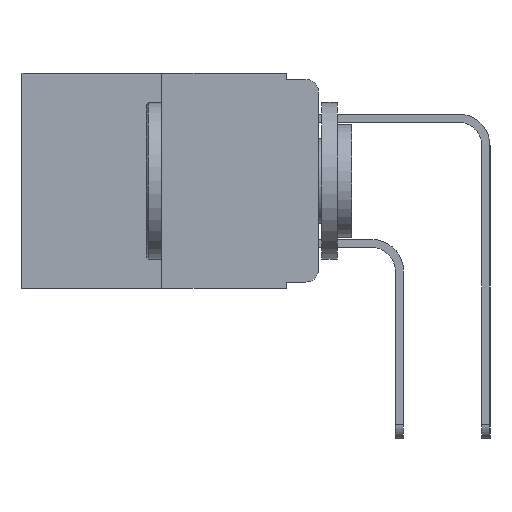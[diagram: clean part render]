
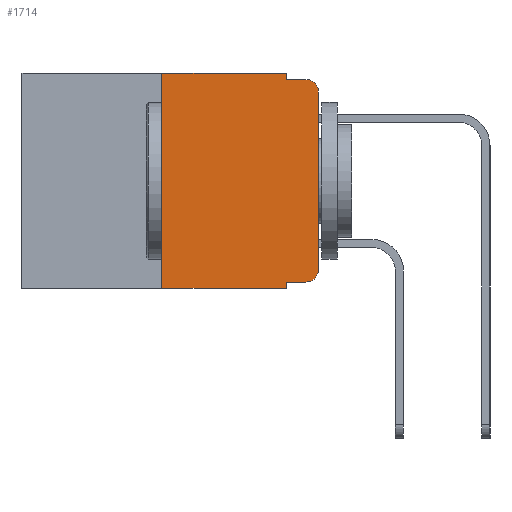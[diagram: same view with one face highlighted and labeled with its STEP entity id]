
A CAD part, left-side view. The second image highlights one B-rep face of the part: STEP entity #1714.
In plain terms, the highlighted planar face has unit normal (-1, 0, 0).
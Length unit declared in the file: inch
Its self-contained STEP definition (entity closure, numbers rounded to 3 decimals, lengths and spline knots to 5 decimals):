
#1017 = VERTEX_POINT ( 'NONE', #15963 ) ;
#1200 = LINE ( 'NONE', #21345, #18734 ) ;
#1714 = ADVANCED_FACE ( 'NONE', ( #17497 ), #11822, .F. ) ;
#1835 = AXIS2_PLACEMENT_3D ( 'NONE', #11015, #10094, #11065 ) ;
#1918 = VERTEX_POINT ( 'NONE', #8275 ) ;
#2695 = VERTEX_POINT ( 'NONE', #4672 ) ;
#2706 = CARTESIAN_POINT ( 'NONE',  ( 0., 0.473, 0. ) ) ;
#2794 = VERTEX_POINT ( 'NONE', #3495 ) ;
#2988 = AXIS2_PLACEMENT_3D ( 'NONE', #6058, #17907, #7817 ) ;
#3069 = CIRCLE ( 'NONE', #2988, 0.02 ) ;
#3096 = EDGE_CURVE ( 'NONE', #1918, #1017, #21475, .T. ) ;
#3413 = LINE ( 'NONE', #7928, #20769 ) ;
#3495 = CARTESIAN_POINT ( 'NONE',  ( 0., 0.051, -0.01 ) ) ;
#3724 = DIRECTION ( 'NONE',  ( 0., -1., 0. ) ) ;
#3997 = LINE ( 'NONE', #19282, #12645 ) ;
#4003 = DIRECTION ( 'NONE',  ( 0., 0., -1. ) ) ;
#4215 = LINE ( 'NONE', #12328, #17250 ) ;
#4513 = DIRECTION ( 'NONE',  ( 0., -1., 0. ) ) ;
#4614 = DIRECTION ( 'NONE',  ( 0., 0., -1. ) ) ;
#4672 = CARTESIAN_POINT ( 'NONE',  ( 0., 0.02, -0.01 ) ) ;
#4783 = ORIENTED_EDGE ( 'NONE', *, *, #11661, .T. ) ;
#4968 = VERTEX_POINT ( 'NONE', #19888 ) ;
#6058 = CARTESIAN_POINT ( 'NONE',  ( 0., 0.02, -0.313 ) ) ;
#6405 = EDGE_CURVE ( 'NONE', #2794, #2695, #3997, .T. ) ;
#6433 = DIRECTION ( 'NONE',  ( 0., 0., -1. ) ) ;
#6610 = CARTESIAN_POINT ( 'NONE',  ( 0., 0.25, 0. ) ) ;
#6652 = ORIENTED_EDGE ( 'NONE', *, *, #21400, .F. ) ;
#7103 = CARTESIAN_POINT ( 'NONE',  ( 0., 0., 0. ) ) ;
#7124 = LINE ( 'NONE', #2706, #15639 ) ;
#7354 = VERTEX_POINT ( 'NONE', #6610 ) ;
#7569 = EDGE_CURVE ( 'NONE', #4968, #2695, #11796, .T. ) ;
#7726 = CARTESIAN_POINT ( 'NONE',  ( 0., 0.02, -0.03 ) ) ;
#7817 = DIRECTION ( 'NONE',  ( 0., 0., -1. ) ) ;
#7851 = VERTEX_POINT ( 'NONE', #21377 ) ;
#7922 = DIRECTION ( 'NONE',  ( -1., 0., 0. ) ) ;
#7928 = CARTESIAN_POINT ( 'NONE',  ( 0., 0.25, 0. ) ) ;
#8275 = CARTESIAN_POINT ( 'NONE',  ( 0., 0.051, -0.333 ) ) ;
#8806 = EDGE_CURVE ( 'NONE', #9960, #4968, #21808, .T. ) ;
#9518 = VERTEX_POINT ( 'NONE', #12397 ) ;
#9570 = CARTESIAN_POINT ( 'NONE',  ( 0., 0.051, -0.343 ) ) ;
#9960 = VERTEX_POINT ( 'NONE', #18775 ) ;
#10030 = ORIENTED_EDGE ( 'NONE', *, *, #8806, .T. ) ;
#10094 = DIRECTION ( 'NONE',  ( 1., 0., 0. ) ) ;
#10244 = VERTEX_POINT ( 'NONE', #9570 ) ;
#10997 = VECTOR ( 'NONE', #4003, 39.37008 ) ;
#11015 = CARTESIAN_POINT ( 'NONE',  ( 0., 0.473, 0. ) ) ;
#11065 = DIRECTION ( 'NONE',  ( 0., 0., -1. ) ) ;
#11318 = ORIENTED_EDGE ( 'NONE', *, *, #21614, .F. ) ;
#11661 = EDGE_CURVE ( 'NONE', #1017, #9960, #3069, .T. ) ;
#11796 = CIRCLE ( 'NONE', #18405, 0.02 ) ;
#11822 = PLANE ( 'NONE',  #1835 ) ;
#12198 = DIRECTION ( 'NONE',  ( 0., 0., 1. ) ) ;
#12328 = CARTESIAN_POINT ( 'NONE',  ( 0., 0.473, -0.343 ) ) ;
#12363 = ORIENTED_EDGE ( 'NONE', *, *, #20100, .T. ) ;
#12397 = CARTESIAN_POINT ( 'NONE',  ( 0., 0.25, -0.343 ) ) ;
#12645 = VECTOR ( 'NONE', #20251, 39.37008 ) ;
#12653 = EDGE_CURVE ( 'NONE', #1918, #10244, #1200, .T. ) ;
#13317 = VECTOR ( 'NONE', #15931, 39.37008 ) ;
#14684 = ORIENTED_EDGE ( 'NONE', *, *, #7569, .T. ) ;
#15639 = VECTOR ( 'NONE', #4513, 39.37008 ) ;
#15717 = ORIENTED_EDGE ( 'NONE', *, *, #20348, .F. ) ;
#15931 = DIRECTION ( 'NONE',  ( 0., -1., 0. ) ) ;
#15963 = CARTESIAN_POINT ( 'NONE',  ( 0., 0.02, -0.333 ) ) ;
#16032 = CARTESIAN_POINT ( 'NONE',  ( 0., 0.051, -0.333 ) ) ;
#16358 = DIRECTION ( 'NONE',  ( 0., 0., 1. ) ) ;
#16762 = ORIENTED_EDGE ( 'NONE', *, *, #12653, .F. ) ;
#17250 = VECTOR ( 'NONE', #3724, 39.37008 ) ;
#17497 = FACE_OUTER_BOUND ( 'NONE', #20395, .T. ) ;
#17790 = ORIENTED_EDGE ( 'NONE', *, *, #3096, .T. ) ;
#17907 = DIRECTION ( 'NONE',  ( -1., 0., 0. ) ) ;
#18405 = AXIS2_PLACEMENT_3D ( 'NONE', #7726, #7922, #6433 ) ;
#18734 = VECTOR ( 'NONE', #4614, 39.37008 ) ;
#18775 = CARTESIAN_POINT ( 'NONE',  ( 0., 0., -0.313 ) ) ;
#19058 = ORIENTED_EDGE ( 'NONE', *, *, #6405, .F. ) ;
#19282 = CARTESIAN_POINT ( 'NONE',  ( 0., 0.051, -0.01 ) ) ;
#19742 = LINE ( 'NONE', #20753, #10997 ) ;
#19888 = CARTESIAN_POINT ( 'NONE',  ( 0., 0., -0.03 ) ) ;
#20100 = EDGE_CURVE ( 'NONE', #9518, #10244, #4215, .T. ) ;
#20251 = DIRECTION ( 'NONE',  ( 0., -1., 0. ) ) ;
#20348 = EDGE_CURVE ( 'NONE', #9518, #7354, #3413, .T. ) ;
#20395 = EDGE_LOOP ( 'NONE', ( #10030, #14684, #19058, #6652, #11318, #15717, #12363, #16762, #17790, #4783 ) ) ;
#20753 = CARTESIAN_POINT ( 'NONE',  ( 0., 0.051, 0. ) ) ;
#20769 = VECTOR ( 'NONE', #16358, 39.37008 ) ;
#21297 = VECTOR ( 'NONE', #12198, 39.37008 ) ;
#21345 = CARTESIAN_POINT ( 'NONE',  ( 0., 0.051, 0. ) ) ;
#21377 = CARTESIAN_POINT ( 'NONE',  ( 0., 0.051, 0. ) ) ;
#21400 = EDGE_CURVE ( 'NONE', #7851, #2794, #19742, .T. ) ;
#21475 = LINE ( 'NONE', #16032, #13317 ) ;
#21614 = EDGE_CURVE ( 'NONE', #7354, #7851, #7124, .T. ) ;
#21808 = LINE ( 'NONE', #7103, #21297 ) ;
